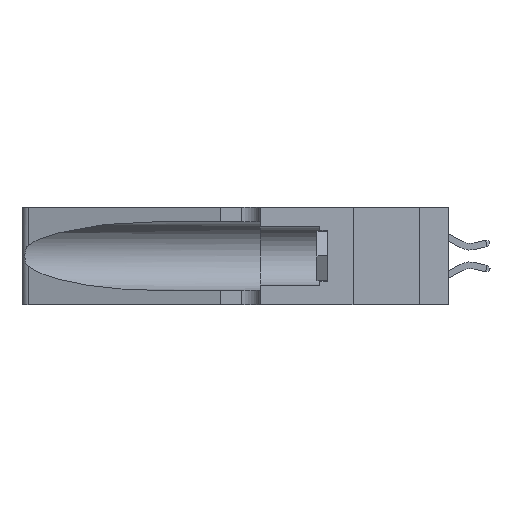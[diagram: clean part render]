
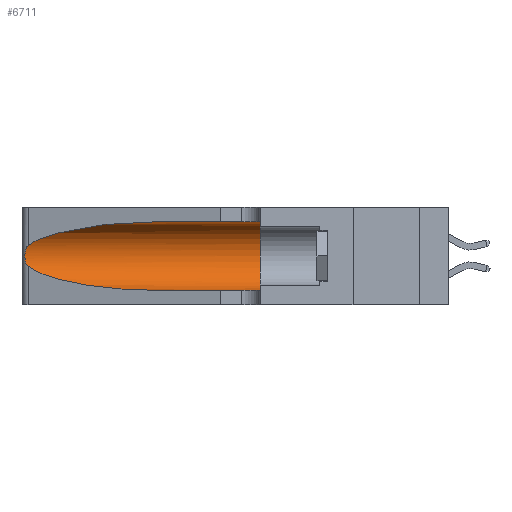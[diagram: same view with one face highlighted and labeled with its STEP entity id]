
A CAD part, left-side view. The second image highlights one B-rep face of the part: STEP entity #6711.
In plain terms, the highlighted cylindrical face has radius 3.308 mm (diameter 6.617 mm), a partial arc.
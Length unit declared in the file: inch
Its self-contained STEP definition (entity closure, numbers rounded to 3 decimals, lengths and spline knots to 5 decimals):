
#255 = CARTESIAN_POINT ( 'NONE',  ( 0.25856, 1.23593, 0.16098 ) ) ;
#392 = VERTEX_POINT ( 'NONE', #905 ) ;
#795 = CARTESIAN_POINT ( 'NONE',  ( 0.25487, 1.22718, 0.14631 ) ) ;
#905 = CARTESIAN_POINT ( 'NONE',  ( 0.1305, 0.72297, 0.31525 ) ) ;
#948 = CARTESIAN_POINT ( 'NONE',  ( 0.25487, 1.22718, 0.22369 ) ) ;
#1080 = VERTEX_POINT ( 'NONE', #948 ) ;
#1245 = CARTESIAN_POINT ( 'NONE',  ( 0.1305, 0.35, 0.185 ) ) ;
#1389 = CARTESIAN_POINT ( 'NONE',  ( 0.25487, 1.22718, 0.22369 ) ) ;
#1565 = DIRECTION ( 'NONE',  ( 0., -1., 0. ) ) ;
#1662 = EDGE_CURVE ( 'NONE', #11336, #3571, #5757, .T. ) ;
#2048 = CARTESIAN_POINT ( 'NONE',  ( 0.25487, 1.22718, 0.14631 ) ) ;
#2147 = CARTESIAN_POINT ( 'NONE',  ( 0.26017, 1.23833, 0.17102 ) ) ;
#2206 = EDGE_CURVE ( 'NONE', #1080, #11336, #5184, .T. ) ;
#2826 = DIRECTION ( 'NONE',  ( 0., 0., 1. ) ) ;
#2957 = VERTEX_POINT ( 'NONE', #11534 ) ;
#3148 = AXIS2_PLACEMENT_3D ( 'NONE', #10732, #1565, #15410 ) ;
#3571 = VERTEX_POINT ( 'NONE', #14887 ) ;
#3742 = EDGE_LOOP ( 'NONE', ( #17306, #6124, #10602, #7085, #14876, #19069 ) ) ;
#3912 = CARTESIAN_POINT ( 'NONE',  ( 0.26075, 1.23896, 0.19203 ) ) ;
#3920 =( BOUNDED_CURVE ( )  B_SPLINE_CURVE ( 3, ( #13911, #9518, #15333, #6550 ),
 .UNSPECIFIED., .F., .F. ) 
 B_SPLINE_CURVE_WITH_KNOTS ( ( 4, 4 ),
 ( 1.5708, 2.84003 ),
 .UNSPECIFIED. ) 
 CURVE ( )  GEOMETRIC_REPRESENTATION_ITEM ( )  RATIONAL_B_SPLINE_CURVE ( ( 1., 0.87, 0.87, 1. ) ) 
 REPRESENTATION_ITEM ( '' )  );
#3932 = EDGE_CURVE ( 'NONE', #9389, #2957, #11291, .T. ) ;
#3942 = CARTESIAN_POINT ( 'NONE',  ( 0.26075, 1.23896, 0.178 ) ) ;
#4095 = VECTOR ( 'NONE', #9378, 39.37008 ) ;
#4423 = CARTESIAN_POINT ( 'NONE',  ( 0.25854, 1.2359, 0.20912 ) ) ;
#4918 = CARTESIAN_POINT ( 'NONE',  ( 0.25555, 1.22993, 0.14849 ) ) ;
#5184 = B_SPLINE_CURVE_WITH_KNOTS ( 'NONE', 3,
 ( #1389, #6533, #13001, #12995, #4423, #12617, #3912, #3942, #2147, #255, #11154, #11822, #4918, #2048 ),
 .UNSPECIFIED., .F., .F.,
 ( 4, 2, 2, 2, 2, 2, 4 ),
 ( 0., 0.00027, 0.00053, 0.00107, 0.0016, 0.00187, 0.00214 ),
 .UNSPECIFIED. ) ;
#5520 = CARTESIAN_POINT ( 'NONE',  ( 0.1305, 1.61858, 0.31525 ) ) ;
#5702 = LINE ( 'NONE', #5520, #9255 ) ;
#5757 =( BOUNDED_CURVE ( )  B_SPLINE_CURVE ( 3, ( #14005, #10388, #6104, #19072 ),
 .UNSPECIFIED., .F., .F. ) 
 B_SPLINE_CURVE_WITH_KNOTS ( ( 4, 4 ),
 ( 3.44316, 4.71239 ),
 .UNSPECIFIED. ) 
 CURVE ( )  GEOMETRIC_REPRESENTATION_ITEM ( )  RATIONAL_B_SPLINE_CURVE ( ( 1., 0.87, 0.87, 1. ) ) 
 REPRESENTATION_ITEM ( '' )  );
#6104 = CARTESIAN_POINT ( 'NONE',  ( 0.18966, 0.96281, 0.05475 ) ) ;
#6117 = EDGE_CURVE ( 'NONE', #392, #1080, #3920, .T. ) ;
#6124 = ORIENTED_EDGE ( 'NONE', *, *, #2206, .T. ) ;
#6531 = FACE_OUTER_BOUND ( 'NONE', #3742, .T. ) ;
#6533 = CARTESIAN_POINT ( 'NONE',  ( 0.25555, 1.22994, 0.2215 ) ) ;
#6550 = CARTESIAN_POINT ( 'NONE',  ( 0.25487, 1.22718, 0.22369 ) ) ;
#6711 = ADVANCED_FACE ( 'NONE', ( #6531 ), #13934, .F. ) ;
#7048 = DIRECTION ( 'NONE',  ( 0., -1., 0. ) ) ;
#7085 = ORIENTED_EDGE ( 'NONE', *, *, #7779, .T. ) ;
#7779 = EDGE_CURVE ( 'NONE', #3571, #2957, #8155, .T. ) ;
#7930 = CARTESIAN_POINT ( 'NONE',  ( 0.1305, 1.61858, 0.05475 ) ) ;
#8155 = LINE ( 'NONE', #7930, #4095 ) ;
#9255 = VECTOR ( 'NONE', #7048, 39.37008 ) ;
#9378 = DIRECTION ( 'NONE',  ( 0., -1., 0. ) ) ;
#9389 = VERTEX_POINT ( 'NONE', #17192 ) ;
#9518 = CARTESIAN_POINT ( 'NONE',  ( 0.18966, 0.96281, 0.31525 ) ) ;
#10388 = CARTESIAN_POINT ( 'NONE',  ( 0.2373, 1.15595, 0.08982 ) ) ;
#10602 = ORIENTED_EDGE ( 'NONE', *, *, #1662, .T. ) ;
#10732 = CARTESIAN_POINT ( 'NONE',  ( 0.1305, 1.61858, 0.185 ) ) ;
#11154 = CARTESIAN_POINT ( 'NONE',  ( 0.25789, 1.23486, 0.15765 ) ) ;
#11291 = CIRCLE ( 'NONE', #18976, 0.13025 ) ;
#11336 = VERTEX_POINT ( 'NONE', #795 ) ;
#11534 = CARTESIAN_POINT ( 'NONE',  ( 0.1305, 0.35, 0.05475 ) ) ;
#11822 = CARTESIAN_POINT ( 'NONE',  ( 0.25639, 1.23186, 0.15144 ) ) ;
#11940 = DIRECTION ( 'NONE',  ( 0., 1., 0. ) ) ;
#12617 = CARTESIAN_POINT ( 'NONE',  ( 0.26018, 1.23835, 0.19895 ) ) ;
#12995 = CARTESIAN_POINT ( 'NONE',  ( 0.25787, 1.23484, 0.2124 ) ) ;
#13001 = CARTESIAN_POINT ( 'NONE',  ( 0.25639, 1.23184, 0.21858 ) ) ;
#13911 = CARTESIAN_POINT ( 'NONE',  ( 0.1305, 0.72297, 0.31525 ) ) ;
#13934 = CYLINDRICAL_SURFACE ( 'NONE', #3148, 0.13025 ) ;
#14005 = CARTESIAN_POINT ( 'NONE',  ( 0.25487, 1.22718, 0.14631 ) ) ;
#14876 = ORIENTED_EDGE ( 'NONE', *, *, #3932, .F. ) ;
#14887 = CARTESIAN_POINT ( 'NONE',  ( 0.1305, 0.72297, 0.05475 ) ) ;
#15333 = CARTESIAN_POINT ( 'NONE',  ( 0.2373, 1.15595, 0.28018 ) ) ;
#15410 = DIRECTION ( 'NONE',  ( 0., 0., -1. ) ) ;
#17192 = CARTESIAN_POINT ( 'NONE',  ( 0.1305, 0.35, 0.31525 ) ) ;
#17306 = ORIENTED_EDGE ( 'NONE', *, *, #6117, .T. ) ;
#17472 = EDGE_CURVE ( 'NONE', #392, #9389, #5702, .T. ) ;
#18976 = AXIS2_PLACEMENT_3D ( 'NONE', #1245, #11940, #2826 ) ;
#19069 = ORIENTED_EDGE ( 'NONE', *, *, #17472, .F. ) ;
#19072 = CARTESIAN_POINT ( 'NONE',  ( 0.1305, 0.72297, 0.05475 ) ) ;
